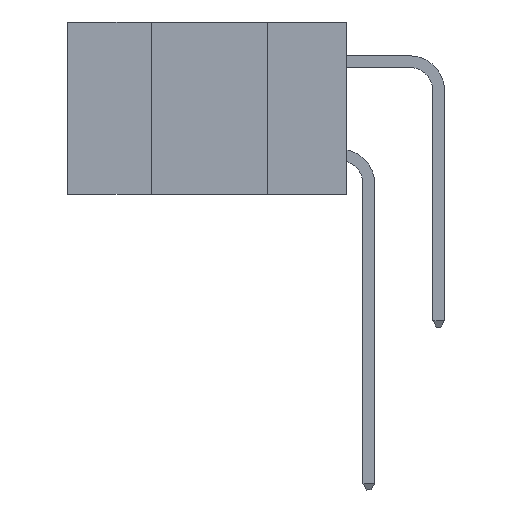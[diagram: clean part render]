
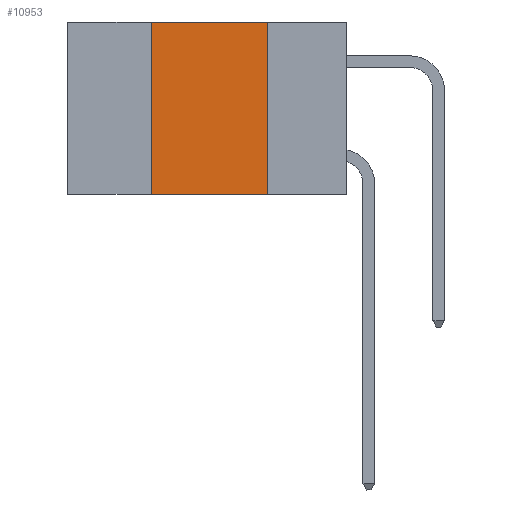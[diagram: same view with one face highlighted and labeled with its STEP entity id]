
A CAD part, left-side view. The second image highlights one B-rep face of the part: STEP entity #10953.
In plain terms, the highlighted planar face has unit normal (-1, 0, 0).
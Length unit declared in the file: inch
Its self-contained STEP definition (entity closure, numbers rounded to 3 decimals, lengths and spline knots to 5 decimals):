
#140 = CARTESIAN_POINT ( 'NONE',  ( 0., 0.6, -0.37 ) ) ;
#211 = LINE ( 'NONE', #7483, #11650 ) ;
#290 = EDGE_CURVE ( 'NONE', #5116, #8686, #8830, .T. ) ;
#530 = ORIENTED_EDGE ( 'NONE', *, *, #290, .F. ) ;
#1218 = PLANE ( 'NONE',  #11899 ) ;
#1261 = EDGE_CURVE ( 'NONE', #6838, #5116, #13264, .T. ) ;
#1374 = DIRECTION ( 'NONE',  ( 0., -1., 0. ) ) ;
#1518 = EDGE_CURVE ( 'NONE', #6838, #13140, #11791, .T. ) ;
#1584 = ORIENTED_EDGE ( 'NONE', *, *, #1261, .F. ) ;
#1900 = DIRECTION ( 'NONE',  ( 0., 0., -1. ) ) ;
#2071 = DIRECTION ( 'NONE',  ( 0., 0., 1. ) ) ;
#2330 = DIRECTION ( 'NONE',  ( 1., 0., 0. ) ) ;
#3190 = CARTESIAN_POINT ( 'NONE',  ( 0., 0.17, -0.37 ) ) ;
#3271 = FACE_OUTER_BOUND ( 'NONE', #9616, .T. ) ;
#3372 = CARTESIAN_POINT ( 'NONE',  ( 0., 0.6, 0. ) ) ;
#4167 = ORIENTED_EDGE ( 'NONE', *, *, #1518, .T. ) ;
#4653 = CARTESIAN_POINT ( 'NONE',  ( 0., 0.42, 0. ) ) ;
#5116 = VERTEX_POINT ( 'NONE', #4653 ) ;
#5517 = CARTESIAN_POINT ( 'NONE',  ( 0., 0.6, 0. ) ) ;
#5853 = VECTOR ( 'NONE', #1374, 39.37008 ) ;
#6499 = ORIENTED_EDGE ( 'NONE', *, *, #12955, .F. ) ;
#6838 = VERTEX_POINT ( 'NONE', #10536 ) ;
#7483 = CARTESIAN_POINT ( 'NONE',  ( 0., 0.17, 0. ) ) ;
#8686 = VERTEX_POINT ( 'NONE', #10114 ) ;
#8830 = LINE ( 'NONE', #5517, #5853 ) ;
#9616 = EDGE_LOOP ( 'NONE', ( #6499, #530, #1584, #4167 ) ) ;
#10114 = CARTESIAN_POINT ( 'NONE',  ( 0., 0.17, 0. ) ) ;
#10127 = DIRECTION ( 'NONE',  ( 0., 0., -1. ) ) ;
#10536 = CARTESIAN_POINT ( 'NONE',  ( 0., 0.42, -0.37 ) ) ;
#10953 = ADVANCED_FACE ( 'NONE', ( #3271 ), #1218, .F. ) ;
#11253 = DIRECTION ( 'NONE',  ( 0., -1., 0. ) ) ;
#11477 = VECTOR ( 'NONE', #11253, 39.37008 ) ;
#11650 = VECTOR ( 'NONE', #1900, 39.37008 ) ;
#11791 = LINE ( 'NONE', #140, #11477 ) ;
#11899 = AXIS2_PLACEMENT_3D ( 'NONE', #3372, #2330, #10127 ) ;
#12604 = CARTESIAN_POINT ( 'NONE',  ( 0., 0.42, 0. ) ) ;
#12955 = EDGE_CURVE ( 'NONE', #8686, #13140, #211, .T. ) ;
#13140 = VERTEX_POINT ( 'NONE', #3190 ) ;
#13264 = LINE ( 'NONE', #12604, #13860 ) ;
#13860 = VECTOR ( 'NONE', #2071, 39.37008 ) ;
